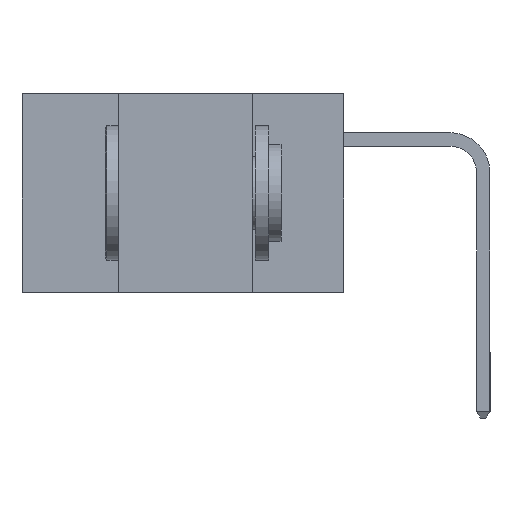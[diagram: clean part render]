
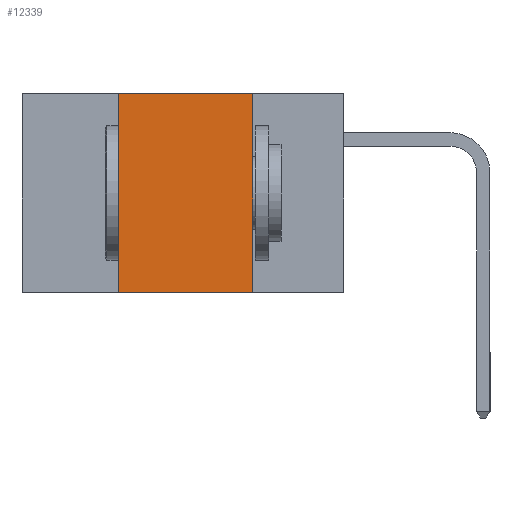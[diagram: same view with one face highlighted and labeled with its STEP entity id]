
A CAD part, left-side view. The second image highlights one B-rep face of the part: STEP entity #12339.
In plain terms, the highlighted planar face has unit normal (-1, 0, 0).
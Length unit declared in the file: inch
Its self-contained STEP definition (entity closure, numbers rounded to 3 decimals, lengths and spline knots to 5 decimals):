
#501 = VERTEX_POINT ( 'NONE', #4426 ) ;
#998 = LINE ( 'NONE', #6949, #4751 ) ;
#1257 = VERTEX_POINT ( 'NONE', #14859 ) ;
#1719 = EDGE_CURVE ( 'NONE', #9132, #4965, #4263, .T. ) ;
#1895 = VECTOR ( 'NONE', #12473, 39.37008 ) ;
#2509 = ORIENTED_EDGE ( 'NONE', *, *, #4002, .F. ) ;
#3282 = DIRECTION ( 'NONE',  ( 1., 0., 0. ) ) ;
#4002 = EDGE_CURVE ( 'NONE', #1257, #501, #8229, .T. ) ;
#4023 = CARTESIAN_POINT ( 'NONE',  ( 0., 0.17, -0.37 ) ) ;
#4263 = LINE ( 'NONE', #8895, #1895 ) ;
#4426 = CARTESIAN_POINT ( 'NONE',  ( 0., 0.42, 0. ) ) ;
#4497 = VECTOR ( 'NONE', #4625, 39.37008 ) ;
#4625 = DIRECTION ( 'NONE',  ( 0., 0., 1. ) ) ;
#4751 = VECTOR ( 'NONE', #6723, 39.37008 ) ;
#4965 = VERTEX_POINT ( 'NONE', #4023 ) ;
#5629 = AXIS2_PLACEMENT_3D ( 'NONE', #15103, #3282, #6712 ) ;
#5657 = ORIENTED_EDGE ( 'NONE', *, *, #15327, .T. ) ;
#6712 = DIRECTION ( 'NONE',  ( 0., 0., -1. ) ) ;
#6723 = DIRECTION ( 'NONE',  ( 0., -1., 0. ) ) ;
#6787 = CARTESIAN_POINT ( 'NONE',  ( 0., 0.42, -0.37 ) ) ;
#6829 = EDGE_CURVE ( 'NONE', #501, #9132, #998, .T. ) ;
#6949 = CARTESIAN_POINT ( 'NONE',  ( 0., 0.6, 0. ) ) ;
#7523 = EDGE_LOOP ( 'NONE', ( #12794, #8531, #2509, #5657 ) ) ;
#8229 = LINE ( 'NONE', #6787, #4497 ) ;
#8531 = ORIENTED_EDGE ( 'NONE', *, *, #6829, .F. ) ;
#8895 = CARTESIAN_POINT ( 'NONE',  ( 0., 0.17, -0.37 ) ) ;
#9132 = VERTEX_POINT ( 'NONE', #11270 ) ;
#9224 = LINE ( 'NONE', #10546, #9490 ) ;
#9490 = VECTOR ( 'NONE', #12945, 39.37008 ) ;
#10546 = CARTESIAN_POINT ( 'NONE',  ( 0., 0.6, -0.37 ) ) ;
#11270 = CARTESIAN_POINT ( 'NONE',  ( 0., 0.17, 0. ) ) ;
#12339 = ADVANCED_FACE ( 'NONE', ( #12743 ), #13853, .F. ) ;
#12473 = DIRECTION ( 'NONE',  ( 0., 0., -1. ) ) ;
#12743 = FACE_OUTER_BOUND ( 'NONE', #7523, .T. ) ;
#12794 = ORIENTED_EDGE ( 'NONE', *, *, #1719, .F. ) ;
#12945 = DIRECTION ( 'NONE',  ( 0., -1., 0. ) ) ;
#13853 = PLANE ( 'NONE',  #5629 ) ;
#14859 = CARTESIAN_POINT ( 'NONE',  ( 0., 0.42, -0.37 ) ) ;
#15103 = CARTESIAN_POINT ( 'NONE',  ( 0., 0.6, 0. ) ) ;
#15327 = EDGE_CURVE ( 'NONE', #1257, #4965, #9224, .T. ) ;
